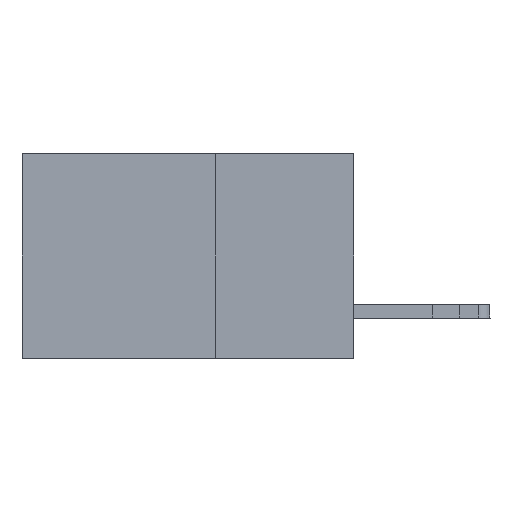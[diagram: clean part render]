
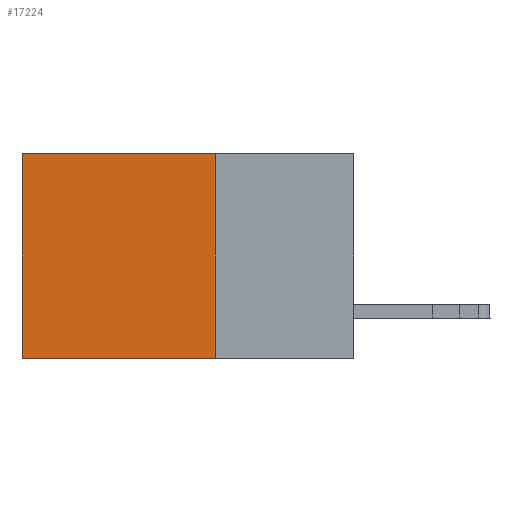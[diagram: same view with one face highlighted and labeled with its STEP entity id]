
A CAD part, left-side view. The second image highlights one B-rep face of the part: STEP entity #17224.
In plain terms, the highlighted planar face has unit normal (-1, 0, 0).
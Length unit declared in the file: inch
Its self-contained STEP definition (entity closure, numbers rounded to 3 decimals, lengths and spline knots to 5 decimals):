
#658 = VERTEX_POINT ( 'NONE', #20981 ) ;
#1377 = CARTESIAN_POINT ( 'NONE',  ( 0.2875, 0.6, 0. ) ) ;
#1379 = LINE ( 'NONE', #29944, #17322 ) ;
#1877 = DIRECTION ( 'NONE',  ( 0., 0., -1. ) ) ;
#4397 = DIRECTION ( 'NONE',  ( 0., 0., -1. ) ) ;
#4887 = DIRECTION ( 'NONE',  ( 1., 0., 0. ) ) ;
#5378 = VECTOR ( 'NONE', #27347, 39.37008 ) ;
#6384 = VECTOR ( 'NONE', #11964, 39.37008 ) ;
#6897 = EDGE_CURVE ( 'NONE', #11009, #658, #7249, .T. ) ;
#7045 = AXIS2_PLACEMENT_3D ( 'NONE', #27747, #4887, #1877 ) ;
#7249 = LINE ( 'NONE', #1377, #29784 ) ;
#9495 = EDGE_CURVE ( 'NONE', #10396, #658, #14962, .T. ) ;
#9731 = EDGE_LOOP ( 'NONE', ( #17112, #12158, #18433, #23773 ) ) ;
#10396 = VERTEX_POINT ( 'NONE', #14879 ) ;
#11009 = VERTEX_POINT ( 'NONE', #28384 ) ;
#11622 = CARTESIAN_POINT ( 'NONE',  ( 0.2875, 0.25, 0. ) ) ;
#11964 = DIRECTION ( 'NONE',  ( 0., 0., -1. ) ) ;
#12158 = ORIENTED_EDGE ( 'NONE', *, *, #9495, .F. ) ;
#12282 = LINE ( 'NONE', #22594, #6384 ) ;
#12509 = VERTEX_POINT ( 'NONE', #11622 ) ;
#14531 = DIRECTION ( 'NONE',  ( 0., 1., 0. ) ) ;
#14879 = CARTESIAN_POINT ( 'NONE',  ( 0.2875, 0.25, -0.37 ) ) ;
#14962 = LINE ( 'NONE', #27998, #5378 ) ;
#17112 = ORIENTED_EDGE ( 'NONE', *, *, #6897, .T. ) ;
#17224 = ADVANCED_FACE ( 'NONE', ( #20268 ), #30601, .F. ) ;
#17322 = VECTOR ( 'NONE', #14531, 39.37008 ) ;
#18433 = ORIENTED_EDGE ( 'NONE', *, *, #25682, .F. ) ;
#20268 = FACE_OUTER_BOUND ( 'NONE', #9731, .T. ) ;
#20981 = CARTESIAN_POINT ( 'NONE',  ( 0.2875, 0.6, -0.37 ) ) ;
#22594 = CARTESIAN_POINT ( 'NONE',  ( 0.2875, 0.25, 0. ) ) ;
#23773 = ORIENTED_EDGE ( 'NONE', *, *, #29941, .T. ) ;
#25682 = EDGE_CURVE ( 'NONE', #12509, #10396, #12282, .T. ) ;
#27347 = DIRECTION ( 'NONE',  ( 0., 1., 0. ) ) ;
#27747 = CARTESIAN_POINT ( 'NONE',  ( 0.2875, 0.25, 0. ) ) ;
#27998 = CARTESIAN_POINT ( 'NONE',  ( 0.2875, 0.25, -0.37 ) ) ;
#28384 = CARTESIAN_POINT ( 'NONE',  ( 0.2875, 0.6, 0. ) ) ;
#29784 = VECTOR ( 'NONE', #4397, 39.37008 ) ;
#29941 = EDGE_CURVE ( 'NONE', #12509, #11009, #1379, .T. ) ;
#29944 = CARTESIAN_POINT ( 'NONE',  ( 0.2875, 0.25, 0. ) ) ;
#30601 = PLANE ( 'NONE',  #7045 ) ;
